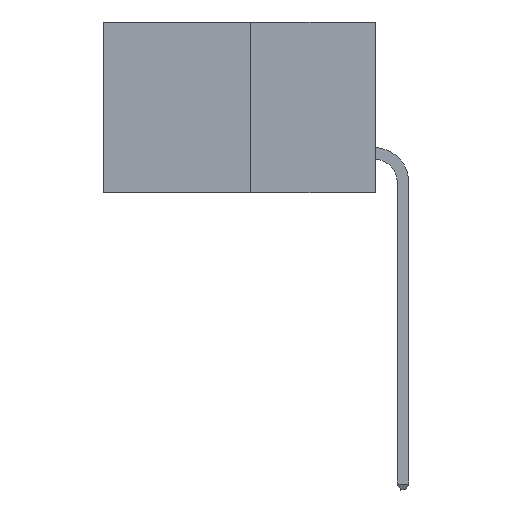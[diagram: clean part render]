
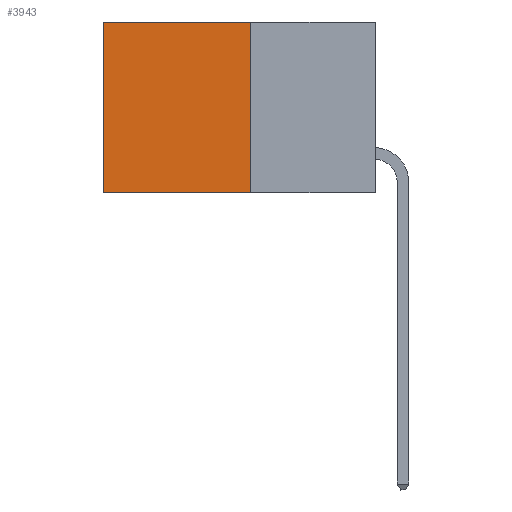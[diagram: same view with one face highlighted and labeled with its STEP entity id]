
A CAD part, left-side view. The second image highlights one B-rep face of the part: STEP entity #3943.
In plain terms, the highlighted planar face has unit normal (-1, 0, 0).
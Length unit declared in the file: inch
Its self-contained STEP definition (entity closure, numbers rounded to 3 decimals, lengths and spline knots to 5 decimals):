
#683 = DIRECTION ( 'NONE',  ( 0., 0., -1. ) ) ;
#1200 = VERTEX_POINT ( 'NONE', #11888 ) ;
#1504 = VECTOR ( 'NONE', #683, 39.37008 ) ;
#1764 = CARTESIAN_POINT ( 'NONE',  ( 0.277, 0.27, -0.37 ) ) ;
#2679 = EDGE_CURVE ( 'NONE', #10814, #1200, #11232, .T. ) ;
#2766 = ORIENTED_EDGE ( 'NONE', *, *, #6576, .T. ) ;
#2824 = VERTEX_POINT ( 'NONE', #5360 ) ;
#3115 = VECTOR ( 'NONE', #4057, 39.37008 ) ;
#3208 = EDGE_LOOP ( 'NONE', ( #6750, #3579, #6352, #2766 ) ) ;
#3227 = VECTOR ( 'NONE', #6386, 39.37008 ) ;
#3579 = ORIENTED_EDGE ( 'NONE', *, *, #2679, .F. ) ;
#3943 = ADVANCED_FACE ( 'NONE', ( #6706 ), #10116, .F. ) ;
#4057 = DIRECTION ( 'NONE',  ( 0., 0., -1. ) ) ;
#4242 = LINE ( 'NONE', #6721, #1504 ) ;
#4361 = DIRECTION ( 'NONE',  ( 1., 0., 0. ) ) ;
#4404 = CARTESIAN_POINT ( 'NONE',  ( 0.277, 0.27, -0.37 ) ) ;
#4674 = CARTESIAN_POINT ( 'NONE',  ( 0.277, 0.27, 0. ) ) ;
#4708 = VECTOR ( 'NONE', #11372, 39.37008 ) ;
#5360 = CARTESIAN_POINT ( 'NONE',  ( 0.277, 0.59, 0. ) ) ;
#6352 = ORIENTED_EDGE ( 'NONE', *, *, #8112, .F. ) ;
#6386 = DIRECTION ( 'NONE',  ( 0., 1., 0. ) ) ;
#6576 = EDGE_CURVE ( 'NONE', #11716, #2824, #9224, .T. ) ;
#6706 = FACE_OUTER_BOUND ( 'NONE', #3208, .T. ) ;
#6721 = CARTESIAN_POINT ( 'NONE',  ( 0.277, 0.59, -0.37 ) ) ;
#6750 = ORIENTED_EDGE ( 'NONE', *, *, #7957, .T. ) ;
#7957 = EDGE_CURVE ( 'NONE', #2824, #1200, #4242, .T. ) ;
#8112 = EDGE_CURVE ( 'NONE', #11716, #10814, #11134, .T. ) ;
#8194 = CARTESIAN_POINT ( 'NONE',  ( 0.277, 0.27, -0.37 ) ) ;
#8217 = AXIS2_PLACEMENT_3D ( 'NONE', #8194, #4361, #11062 ) ;
#8870 = CARTESIAN_POINT ( 'NONE',  ( 0.277, 0.27, -0.37 ) ) ;
#9224 = LINE ( 'NONE', #4674, #4708 ) ;
#10116 = PLANE ( 'NONE',  #8217 ) ;
#10814 = VERTEX_POINT ( 'NONE', #1764 ) ;
#11062 = DIRECTION ( 'NONE',  ( 0., 0., -1. ) ) ;
#11134 = LINE ( 'NONE', #8870, #3115 ) ;
#11172 = CARTESIAN_POINT ( 'NONE',  ( 0.277, 0.27, 0. ) ) ;
#11232 = LINE ( 'NONE', #4404, #3227 ) ;
#11372 = DIRECTION ( 'NONE',  ( 0., 1., 0. ) ) ;
#11716 = VERTEX_POINT ( 'NONE', #11172 ) ;
#11888 = CARTESIAN_POINT ( 'NONE',  ( 0.277, 0.59, -0.37 ) ) ;
